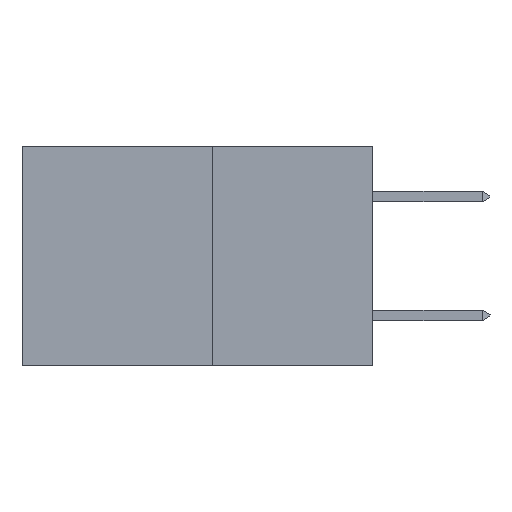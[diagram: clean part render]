
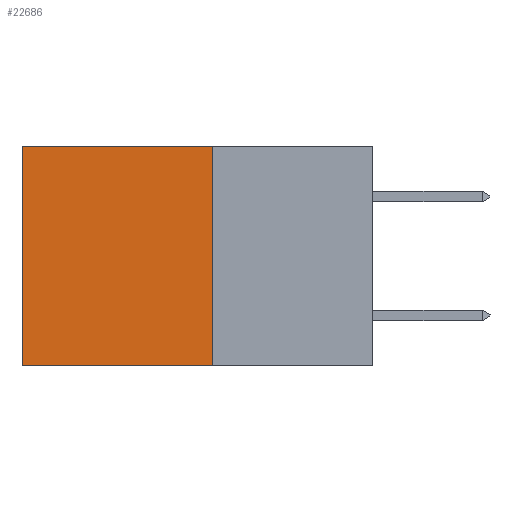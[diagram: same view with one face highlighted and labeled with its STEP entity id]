
A CAD part, left-side view. The second image highlights one B-rep face of the part: STEP entity #22686.
In plain terms, the highlighted planar face has unit normal (-1, 0, 0).
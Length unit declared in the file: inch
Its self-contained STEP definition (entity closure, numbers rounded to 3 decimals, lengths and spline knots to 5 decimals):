
#3707 = DIRECTION ( 'NONE',  ( 0., 1., 0. ) ) ;
#4163 = CARTESIAN_POINT ( 'NONE',  ( 0.277, 0.27, -0.37 ) ) ;
#5004 = CARTESIAN_POINT ( 'NONE',  ( 0.277, 0.59, -0.37 ) ) ;
#5123 = VERTEX_POINT ( 'NONE', #15872 ) ;
#7054 = EDGE_CURVE ( 'NONE', #10157, #5123, #7287, .T. ) ;
#7287 = LINE ( 'NONE', #9603, #18229 ) ;
#7823 = FACE_OUTER_BOUND ( 'NONE', #10496, .T. ) ;
#8097 = PLANE ( 'NONE',  #13093 ) ;
#9603 = CARTESIAN_POINT ( 'NONE',  ( 0.277, 0.27, 0. ) ) ;
#9781 = VECTOR ( 'NONE', #22956, 39.37008 ) ;
#10157 = VERTEX_POINT ( 'NONE', #24828 ) ;
#10496 = EDGE_LOOP ( 'NONE', ( #24683, #14136, #12767, #16338 ) ) ;
#11311 = CARTESIAN_POINT ( 'NONE',  ( 0.277, 0.59, -0.37 ) ) ;
#11997 = DIRECTION ( 'NONE',  ( 0., 0., -1. ) ) ;
#12525 = EDGE_CURVE ( 'NONE', #23278, #13468, #18587, .T. ) ;
#12767 = ORIENTED_EDGE ( 'NONE', *, *, #24532, .F. ) ;
#13093 = AXIS2_PLACEMENT_3D ( 'NONE', #4163, #23640, #11997 ) ;
#13459 = DIRECTION ( 'NONE',  ( 0., 1., 0. ) ) ;
#13468 = VERTEX_POINT ( 'NONE', #5004 ) ;
#13488 = LINE ( 'NONE', #18987, #23233 ) ;
#14136 = ORIENTED_EDGE ( 'NONE', *, *, #12525, .F. ) ;
#14929 = LINE ( 'NONE', #11311, #9781 ) ;
#15794 = EDGE_CURVE ( 'NONE', #5123, #13468, #14929, .T. ) ;
#15872 = CARTESIAN_POINT ( 'NONE',  ( 0.277, 0.59, 0. ) ) ;
#16338 = ORIENTED_EDGE ( 'NONE', *, *, #7054, .T. ) ;
#17974 = VECTOR ( 'NONE', #13459, 39.37008 ) ;
#18229 = VECTOR ( 'NONE', #3707, 39.37008 ) ;
#18587 = LINE ( 'NONE', #19265, #17974 ) ;
#18987 = CARTESIAN_POINT ( 'NONE',  ( 0.277, 0.27, -0.37 ) ) ;
#19265 = CARTESIAN_POINT ( 'NONE',  ( 0.277, 0.27, -0.37 ) ) ;
#20964 = DIRECTION ( 'NONE',  ( 0., 0., -1. ) ) ;
#22686 = ADVANCED_FACE ( 'NONE', ( #7823 ), #8097, .F. ) ;
#22956 = DIRECTION ( 'NONE',  ( 0., 0., -1. ) ) ;
#23233 = VECTOR ( 'NONE', #20964, 39.37008 ) ;
#23278 = VERTEX_POINT ( 'NONE', #23355 ) ;
#23355 = CARTESIAN_POINT ( 'NONE',  ( 0.277, 0.27, -0.37 ) ) ;
#23640 = DIRECTION ( 'NONE',  ( 1., 0., 0. ) ) ;
#24532 = EDGE_CURVE ( 'NONE', #10157, #23278, #13488, .T. ) ;
#24683 = ORIENTED_EDGE ( 'NONE', *, *, #15794, .T. ) ;
#24828 = CARTESIAN_POINT ( 'NONE',  ( 0.277, 0.27, 0. ) ) ;
